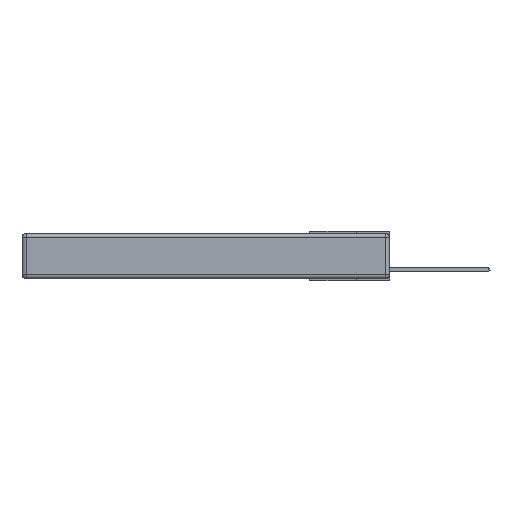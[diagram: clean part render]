
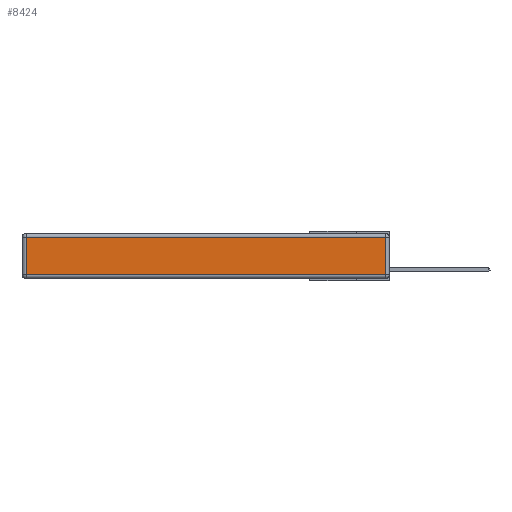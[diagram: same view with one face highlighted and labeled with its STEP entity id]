
A CAD part, left-side view. The second image highlights one B-rep face of the part: STEP entity #8424.
In plain terms, the highlighted planar face has unit normal (-1, 0, 0).
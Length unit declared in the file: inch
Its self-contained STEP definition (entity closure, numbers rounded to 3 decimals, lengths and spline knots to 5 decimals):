
#713 = CARTESIAN_POINT ( 'NONE',  ( 0., 2.72, -0.313 ) ) ;
#856 = ORIENTED_EDGE ( 'NONE', *, *, #24112, .T. ) ;
#1220 = ORIENTED_EDGE ( 'NONE', *, *, #23918, .T. ) ;
#1330 = ORIENTED_EDGE ( 'NONE', *, *, #5840, .T. ) ;
#1715 = DIRECTION ( 'NONE',  ( 0., -1., 0. ) ) ;
#1849 = ORIENTED_EDGE ( 'NONE', *, *, #19782, .T. ) ;
#3075 = LINE ( 'NONE', #8658, #10242 ) ;
#3654 = PLANE ( 'NONE',  #17229 ) ;
#5600 = CARTESIAN_POINT ( 'NONE',  ( 0., 0., -0.343 ) ) ;
#5840 = EDGE_CURVE ( 'NONE', #10490, #23484, #7242, .T. ) ;
#6333 = EDGE_LOOP ( 'NONE', ( #1330, #1849, #1220, #856 ) ) ;
#6443 = DIRECTION ( 'NONE',  ( 0., 0., -1. ) ) ;
#6969 = LINE ( 'NONE', #23061, #20063 ) ;
#7242 = LINE ( 'NONE', #19205, #13130 ) ;
#8068 = CARTESIAN_POINT ( 'NONE',  ( 0., 0.03, -0.313 ) ) ;
#8424 = ADVANCED_FACE ( 'NONE', ( #24302 ), #3654, .T. ) ;
#8658 = CARTESIAN_POINT ( 'NONE',  ( 0., 2.72, -0.343 ) ) ;
#10242 = VECTOR ( 'NONE', #6443, 39.37008 ) ;
#10490 = VERTEX_POINT ( 'NONE', #713 ) ;
#10524 = CARTESIAN_POINT ( 'NONE',  ( 0., 0.03, -0.343 ) ) ;
#10609 = CARTESIAN_POINT ( 'NONE',  ( 0., 0.03, -0.03 ) ) ;
#12265 = VERTEX_POINT ( 'NONE', #10609 ) ;
#13130 = VECTOR ( 'NONE', #1715, 39.37008 ) ;
#13447 = LINE ( 'NONE', #10524, #24414 ) ;
#17023 = CARTESIAN_POINT ( 'NONE',  ( 0., 2.72, -0.03 ) ) ;
#17132 = DIRECTION ( 'NONE',  ( -1., 0., 0. ) ) ;
#17178 = DIRECTION ( 'NONE',  ( 0., 1., 0. ) ) ;
#17229 = AXIS2_PLACEMENT_3D ( 'NONE', #5600, #17132, #20613 ) ;
#18086 = DIRECTION ( 'NONE',  ( 0., 0., 1. ) ) ;
#19205 = CARTESIAN_POINT ( 'NONE',  ( 0., 0., -0.313 ) ) ;
#19469 = VERTEX_POINT ( 'NONE', #17023 ) ;
#19782 = EDGE_CURVE ( 'NONE', #23484, #12265, #13447, .T. ) ;
#20063 = VECTOR ( 'NONE', #17178, 39.37008 ) ;
#20613 = DIRECTION ( 'NONE',  ( 0., 0., 1. ) ) ;
#23061 = CARTESIAN_POINT ( 'NONE',  ( 0., 2.75, -0.03 ) ) ;
#23484 = VERTEX_POINT ( 'NONE', #8068 ) ;
#23918 = EDGE_CURVE ( 'NONE', #12265, #19469, #6969, .T. ) ;
#24112 = EDGE_CURVE ( 'NONE', #19469, #10490, #3075, .T. ) ;
#24302 = FACE_OUTER_BOUND ( 'NONE', #6333, .T. ) ;
#24414 = VECTOR ( 'NONE', #18086, 39.37008 ) ;
